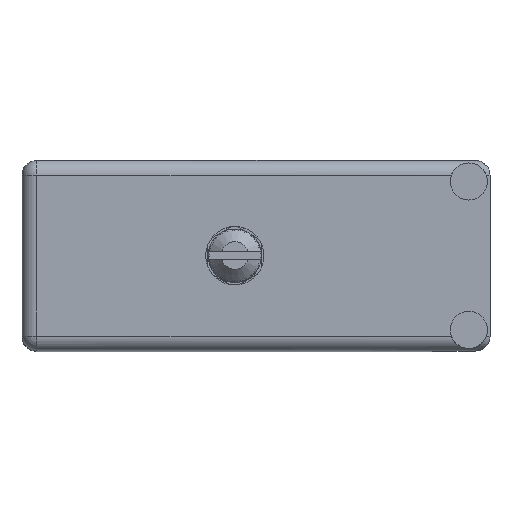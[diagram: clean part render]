
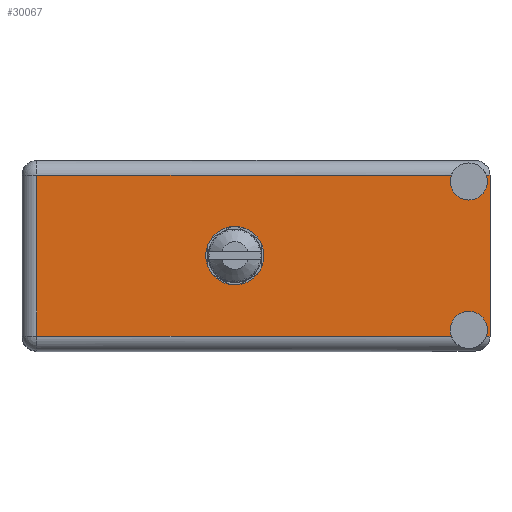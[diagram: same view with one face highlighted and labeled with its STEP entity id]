
A CAD part, top view. The second image highlights one B-rep face of the part: STEP entity #30067.
In plain terms, the highlighted face is planar.
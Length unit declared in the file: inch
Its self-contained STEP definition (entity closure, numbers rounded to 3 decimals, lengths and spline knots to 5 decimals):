
#253 = DIRECTION ( 'NONE',  ( -1., 0., 0. ) ) ;
#1995 = CARTESIAN_POINT ( 'NONE',  ( 1.004, 1.566, -0.4495 ) ) ;
#6554 = ORIENTED_EDGE ( 'NONE', *, *, #15347, .F. ) ;
#7639 = DIRECTION ( 'NONE',  ( 1., 0., 0. ) ) ;
#7649 = DIRECTION ( 'NONE',  ( 0., 0., 1. ) ) ;
#8805 = CARTESIAN_POINT ( 'NONE',  ( 2.108, 1.566, -0.0995 ) ) ;
#9472 = CARTESIAN_POINT ( 'NONE',  ( 1.004, 1.566, -0.312 ) ) ;
#11040 = ORIENTED_EDGE ( 'NONE', *, *, #28106, .F. ) ;
#12917 = DIRECTION ( 'NONE',  ( 0., 0., 1. ) ) ;
#13152 = VECTOR ( 'NONE', #7639, 39.37008 ) ;
#13514 = CIRCLE ( 'NONE', #63943, 0.0875 ) ;
#14094 = CARTESIAN_POINT ( 'NONE',  ( 2.208, 1.566, -0.07 ) ) ;
#14421 = ORIENTED_EDGE ( 'NONE', *, *, #92295, .T. ) ;
#15347 = EDGE_CURVE ( 'NONE', #24771, #50534, #83285, .T. ) ;
#16019 = ORIENTED_EDGE ( 'NONE', *, *, #61918, .F. ) ;
#17472 = CARTESIAN_POINT ( 'NONE',  ( 2.208, 1.566, -0.829 ) ) ;
#18499 = ORIENTED_EDGE ( 'NONE', *, *, #53615, .T. ) ;
#18730 = ORIENTED_EDGE ( 'NONE', *, *, #34032, .F. ) ;
#20205 = ORIENTED_EDGE ( 'NONE', *, *, #55538, .F. ) ;
#21361 = DIRECTION ( 'NONE',  ( 0., 1., 0. ) ) ;
#21370 = VERTEX_POINT ( 'NONE', #34591 ) ;
#21961 = CARTESIAN_POINT ( 'NONE',  ( 2.19038, 1.566, -0.07 ) ) ;
#23616 = VECTOR ( 'NONE', #84252, 39.37008 ) ;
#23815 = CIRCLE ( 'NONE', #82697, 0.0875 ) ;
#24054 = EDGE_CURVE ( 'NONE', #49545, #89656, #48140, .T. ) ;
#24595 = DIRECTION ( 'NONE',  ( 0., 0., 1. ) ) ;
#24771 = VERTEX_POINT ( 'NONE', #58291 ) ;
#25099 = EDGE_CURVE ( 'NONE', #21370, #26468, #88228, .T. ) ;
#26450 = ORIENTED_EDGE ( 'NONE', *, *, #24054, .T. ) ;
#26468 = VERTEX_POINT ( 'NONE', #74272 ) ;
#26720 = EDGE_CURVE ( 'NONE', #104064, #45606, #65186, .T. ) ;
#26887 = CARTESIAN_POINT ( 'NONE',  ( 0., 1.566, -0.899 ) ) ;
#27144 = VECTOR ( 'NONE', #37820, 39.37008 ) ;
#27585 = VERTEX_POINT ( 'NONE', #30014 ) ;
#28106 = EDGE_CURVE ( 'NONE', #67558, #89656, #23815, .T. ) ;
#29237 = CARTESIAN_POINT ( 'NONE',  ( 2.19038, 1.566, -0.829 ) ) ;
#30014 = CARTESIAN_POINT ( 'NONE',  ( 2.208, 1.566, -0.07 ) ) ;
#30067 = ADVANCED_FACE ( 'NONE', ( #92749, #34805 ), #67958, .T. ) ;
#31308 = CARTESIAN_POINT ( 'NONE',  ( 2.108, 1.566, -0.7995 ) ) ;
#31458 = LINE ( 'NONE', #14094, #27144 ) ;
#32887 = AXIS2_PLACEMENT_3D ( 'NONE', #57421, #49499, #48982 ) ;
#34032 = EDGE_CURVE ( 'NONE', #104064, #67558, #47978, .T. ) ;
#34181 = ORIENTED_EDGE ( 'NONE', *, *, #25099, .T. ) ;
#34591 = CARTESIAN_POINT ( 'NONE',  ( 0.07, 1.566, -0.07 ) ) ;
#34805 = FACE_OUTER_BOUND ( 'NONE', #57572, .T. ) ;
#35326 = DIRECTION ( 'NONE',  ( 0., 0., 1. ) ) ;
#36873 = DIRECTION ( 'NONE',  ( 0., 1., 0. ) ) ;
#37820 = DIRECTION ( 'NONE',  ( 1., 0., 0. ) ) ;
#38797 = VERTEX_POINT ( 'NONE', #72499 ) ;
#40922 = DIRECTION ( 'NONE',  ( 0., 1., 0. ) ) ;
#42539 = DIRECTION ( 'NONE',  ( 0., 0., 1. ) ) ;
#45214 = ORIENTED_EDGE ( 'NONE', *, *, #60533, .F. ) ;
#45606 = VERTEX_POINT ( 'NONE', #88200 ) ;
#47647 = CARTESIAN_POINT ( 'NONE',  ( 1.004, 1.566, -0.4495 ) ) ;
#47978 = CIRCLE ( 'NONE', #32887, 0.0875 ) ;
#48140 = LINE ( 'NONE', #65517, #63571 ) ;
#48906 = AXIS2_PLACEMENT_3D ( 'NONE', #26887, #36873, #35326 ) ;
#48982 = DIRECTION ( 'NONE',  ( 0., 0., 1. ) ) ;
#49499 = DIRECTION ( 'NONE',  ( 0., 1., 0. ) ) ;
#49545 = VERTEX_POINT ( 'NONE', #17472 ) ;
#50534 = VERTEX_POINT ( 'NONE', #9472 ) ;
#53615 = EDGE_CURVE ( 'NONE', #45606, #21370, #60510, .T. ) ;
#53653 = CARTESIAN_POINT ( 'NONE',  ( 0.07, 1.566, -0.899 ) ) ;
#55538 = EDGE_CURVE ( 'NONE', #49545, #27585, #95457, .T. ) ;
#55612 = AXIS2_PLACEMENT_3D ( 'NONE', #1995, #99473, #42539 ) ;
#56252 = DIRECTION ( 'NONE',  ( -1., 0., 0. ) ) ;
#56338 = AXIS2_PLACEMENT_3D ( 'NONE', #47647, #103056, #7649 ) ;
#57421 = CARTESIAN_POINT ( 'NONE',  ( 2.108, 1.566, -0.7995 ) ) ;
#57572 = EDGE_LOOP ( 'NONE', ( #34181, #45214, #68127, #14421, #20205, #26450, #11040, #18730, #72061, #18499 ) ) ;
#58291 = CARTESIAN_POINT ( 'NONE',  ( 1.004, 1.566, -0.587 ) ) ;
#60510 = LINE ( 'NONE', #53653, #23616 ) ;
#60533 = EDGE_CURVE ( 'NONE', #38797, #26468, #13514, .T. ) ;
#60727 = CIRCLE ( 'NONE', #55612, 0.1375 ) ;
#61188 = DIRECTION ( 'NONE',  ( 0., 1., 0. ) ) ;
#61918 = EDGE_CURVE ( 'NONE', #50534, #24771, #60727, .T. ) ;
#63571 = VECTOR ( 'NONE', #253, 39.37008 ) ;
#63915 = CIRCLE ( 'NONE', #72353, 0.0875 ) ;
#63943 = AXIS2_PLACEMENT_3D ( 'NONE', #8805, #40922, #24595 ) ;
#65186 = LINE ( 'NONE', #65715, #88821 ) ;
#65517 = CARTESIAN_POINT ( 'NONE',  ( 0., 1.566, -0.829 ) ) ;
#65715 = CARTESIAN_POINT ( 'NONE',  ( 0., 1.566, -0.829 ) ) ;
#67558 = VERTEX_POINT ( 'NONE', #103577 ) ;
#67958 = PLANE ( 'NONE',  #48906 ) ;
#68127 = ORIENTED_EDGE ( 'NONE', *, *, #68961, .F. ) ;
#68961 = EDGE_CURVE ( 'NONE', #75615, #38797, #63915, .T. ) ;
#72061 = ORIENTED_EDGE ( 'NONE', *, *, #26720, .T. ) ;
#72353 = AXIS2_PLACEMENT_3D ( 'NONE', #87511, #61188, #78024 ) ;
#72499 = CARTESIAN_POINT ( 'NONE',  ( 2.108, 1.566, -0.187 ) ) ;
#74272 = CARTESIAN_POINT ( 'NONE',  ( 2.02562, 1.566, -0.07 ) ) ;
#75615 = VERTEX_POINT ( 'NONE', #21961 ) ;
#78024 = DIRECTION ( 'NONE',  ( 0., 0., 1. ) ) ;
#79049 = EDGE_LOOP ( 'NONE', ( #16019, #6554 ) ) ;
#82697 = AXIS2_PLACEMENT_3D ( 'NONE', #31308, #21361, #12917 ) ;
#83285 = CIRCLE ( 'NONE', #56338, 0.1375 ) ;
#84252 = DIRECTION ( 'NONE',  ( 0., 0., 1. ) ) ;
#87511 = CARTESIAN_POINT ( 'NONE',  ( 2.108, 1.566, -0.0995 ) ) ;
#88200 = CARTESIAN_POINT ( 'NONE',  ( 0.07, 1.566, -0.829 ) ) ;
#88228 = LINE ( 'NONE', #96166, #13152 ) ;
#88821 = VECTOR ( 'NONE', #56252, 39.37008 ) ;
#89656 = VERTEX_POINT ( 'NONE', #29237 ) ;
#92295 = EDGE_CURVE ( 'NONE', #75615, #27585, #31458, .T. ) ;
#92749 = FACE_BOUND ( 'NONE', #79049, .T. ) ;
#94328 = VECTOR ( 'NONE', #103891, 39.37008 ) ;
#95457 = LINE ( 'NONE', #102864, #94328 ) ;
#96166 = CARTESIAN_POINT ( 'NONE',  ( 2.208, 1.566, -0.07 ) ) ;
#99084 = CARTESIAN_POINT ( 'NONE',  ( 2.02562, 1.566, -0.829 ) ) ;
#99473 = DIRECTION ( 'NONE',  ( 0., 1., 0. ) ) ;
#102864 = CARTESIAN_POINT ( 'NONE',  ( 2.208, 1.566, 0. ) ) ;
#103056 = DIRECTION ( 'NONE',  ( 0., 1., 0. ) ) ;
#103577 = CARTESIAN_POINT ( 'NONE',  ( 2.108, 1.566, -0.712 ) ) ;
#103891 = DIRECTION ( 'NONE',  ( 0., 0., 1. ) ) ;
#104064 = VERTEX_POINT ( 'NONE', #99084 ) ;
